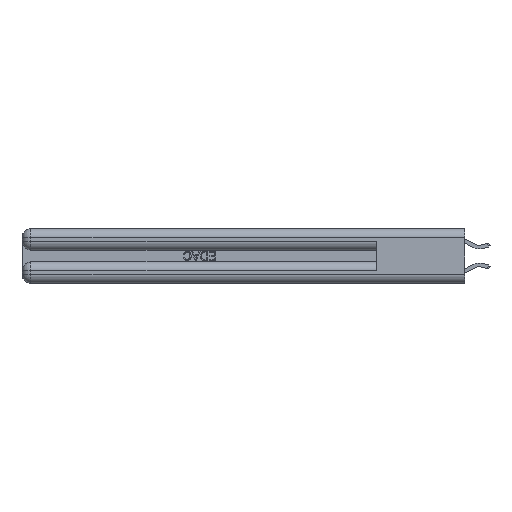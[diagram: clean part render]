
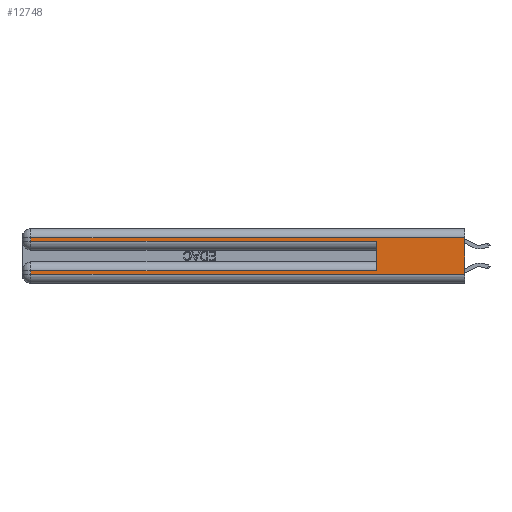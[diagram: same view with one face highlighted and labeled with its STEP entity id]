
A CAD part, left-side view. The second image highlights one B-rep face of the part: STEP entity #12748.
In plain terms, the highlighted planar face has unit normal (-1, 0, 0).
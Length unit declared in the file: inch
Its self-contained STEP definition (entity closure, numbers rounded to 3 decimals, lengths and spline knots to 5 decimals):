
#625 = VECTOR ( 'NONE', #8974, 39.37008 ) ;
#682 = CARTESIAN_POINT ( 'NONE',  ( 0., 0., 0.06 ) ) ;
#769 = LINE ( 'NONE', #8257, #14219 ) ;
#927 = CARTESIAN_POINT ( 'NONE',  ( 0., 0., 0.31 ) ) ;
#1023 = ORIENTED_EDGE ( 'NONE', *, *, #10449, .F. ) ;
#1034 = DIRECTION ( 'NONE',  ( 0., 1., 0. ) ) ;
#1046 = VERTEX_POINT ( 'NONE', #682 ) ;
#3208 = CARTESIAN_POINT ( 'NONE',  ( 0., 2.94, 0.285 ) ) ;
#3388 = LINE ( 'NONE', #22366, #15110 ) ;
#4295 = ORIENTED_EDGE ( 'NONE', *, *, #7782, .T. ) ;
#4301 = ORIENTED_EDGE ( 'NONE', *, *, #24317, .F. ) ;
#4869 = VECTOR ( 'NONE', #25809, 39.37008 ) ;
#5578 = DIRECTION ( 'NONE',  ( 0., 0., -1. ) ) ;
#5681 = AXIS2_PLACEMENT_3D ( 'NONE', #17427, #28870, #5578 ) ;
#5893 = ORIENTED_EDGE ( 'NONE', *, *, #7988, .T. ) ;
#6182 = DIRECTION ( 'NONE',  ( 0., 0., -1. ) ) ;
#6501 = VERTEX_POINT ( 'NONE', #30517 ) ;
#7486 = CARTESIAN_POINT ( 'NONE',  ( 0., 2.94, 0.06 ) ) ;
#7652 = VECTOR ( 'NONE', #6182, 39.37008 ) ;
#7674 = EDGE_CURVE ( 'NONE', #6501, #16343, #19790, .T. ) ;
#7782 = EDGE_CURVE ( 'NONE', #16343, #11686, #769, .T. ) ;
#7988 = EDGE_CURVE ( 'NONE', #11686, #28070, #16170, .T. ) ;
#8257 = CARTESIAN_POINT ( 'NONE',  ( 0., 2.94, 0.37 ) ) ;
#8302 = VECTOR ( 'NONE', #16791, 39.37008 ) ;
#8974 = DIRECTION ( 'NONE',  ( 0., 0., 1. ) ) ;
#9316 = CARTESIAN_POINT ( 'NONE',  ( 0., 0., 0.285 ) ) ;
#9434 = CARTESIAN_POINT ( 'NONE',  ( 0., 0.6, 0.145 ) ) ;
#9479 = ORIENTED_EDGE ( 'NONE', *, *, #20115, .T. ) ;
#9810 = VERTEX_POINT ( 'NONE', #7486 ) ;
#9968 = ORIENTED_EDGE ( 'NONE', *, *, #27296, .T. ) ;
#9981 = VERTEX_POINT ( 'NONE', #11053 ) ;
#10273 = VERTEX_POINT ( 'NONE', #19905 ) ;
#10449 = EDGE_CURVE ( 'NONE', #9981, #28070, #28219, .T. ) ;
#10872 = CARTESIAN_POINT ( 'NONE',  ( 0., 2.94, 0.37 ) ) ;
#11053 = CARTESIAN_POINT ( 'NONE',  ( 0., 0.6, 0.085 ) ) ;
#11686 = VERTEX_POINT ( 'NONE', #3208 ) ;
#12748 = ADVANCED_FACE ( 'NONE', ( #17119 ), #24092, .F. ) ;
#12854 = EDGE_CURVE ( 'NONE', #10273, #9810, #13205, .T. ) ;
#13205 = LINE ( 'NONE', #10872, #7652 ) ;
#14183 = LINE ( 'NONE', #30606, #4869 ) ;
#14219 = VECTOR ( 'NONE', #29205, 39.37008 ) ;
#14267 = LINE ( 'NONE', #16428, #15772 ) ;
#15110 = VECTOR ( 'NONE', #1034, 39.37008 ) ;
#15772 = VECTOR ( 'NONE', #16758, 39.37008 ) ;
#16170 = LINE ( 'NONE', #9316, #8302 ) ;
#16343 = VERTEX_POINT ( 'NONE', #16363 ) ;
#16363 = CARTESIAN_POINT ( 'NONE',  ( 0., 2.94, 0.31 ) ) ;
#16428 = CARTESIAN_POINT ( 'NONE',  ( 0., 0., 0.37 ) ) ;
#16758 = DIRECTION ( 'NONE',  ( 0., 0., -1. ) ) ;
#16791 = DIRECTION ( 'NONE',  ( 0., -1., 0. ) ) ;
#17119 = FACE_OUTER_BOUND ( 'NONE', #21047, .T. ) ;
#17427 = CARTESIAN_POINT ( 'NONE',  ( 0., 0., 0.37 ) ) ;
#19203 = VECTOR ( 'NONE', #29504, 39.37008 ) ;
#19790 = LINE ( 'NONE', #927, #19203 ) ;
#19905 = CARTESIAN_POINT ( 'NONE',  ( 0., 2.94, 0.085 ) ) ;
#20115 = EDGE_CURVE ( 'NONE', #9981, #10273, #3388, .T. ) ;
#20830 = ORIENTED_EDGE ( 'NONE', *, *, #7674, .T. ) ;
#21047 = EDGE_LOOP ( 'NONE', ( #4301, #20830, #4295, #5893, #1023, #9479, #28475, #9968 ) ) ;
#22366 = CARTESIAN_POINT ( 'NONE',  ( 0., 0., 0.085 ) ) ;
#23081 = CARTESIAN_POINT ( 'NONE',  ( 0., 0.6, 0.285 ) ) ;
#24092 = PLANE ( 'NONE',  #5681 ) ;
#24317 = EDGE_CURVE ( 'NONE', #6501, #1046, #14267, .T. ) ;
#25809 = DIRECTION ( 'NONE',  ( 0., -1., 0. ) ) ;
#27296 = EDGE_CURVE ( 'NONE', #9810, #1046, #14183, .T. ) ;
#28070 = VERTEX_POINT ( 'NONE', #23081 ) ;
#28219 = LINE ( 'NONE', #9434, #625 ) ;
#28475 = ORIENTED_EDGE ( 'NONE', *, *, #12854, .T. ) ;
#28870 = DIRECTION ( 'NONE',  ( 1., 0., 0. ) ) ;
#29205 = DIRECTION ( 'NONE',  ( 0., 0., -1. ) ) ;
#29504 = DIRECTION ( 'NONE',  ( 0., 1., 0. ) ) ;
#30517 = CARTESIAN_POINT ( 'NONE',  ( 0., 0., 0.31 ) ) ;
#30606 = CARTESIAN_POINT ( 'NONE',  ( 0., 0., 0.06 ) ) ;
